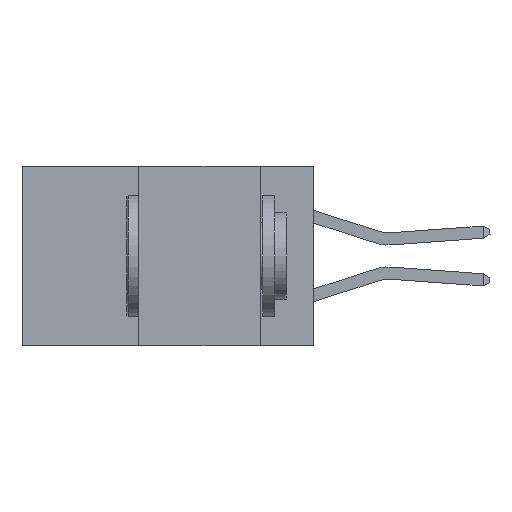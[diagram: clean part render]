
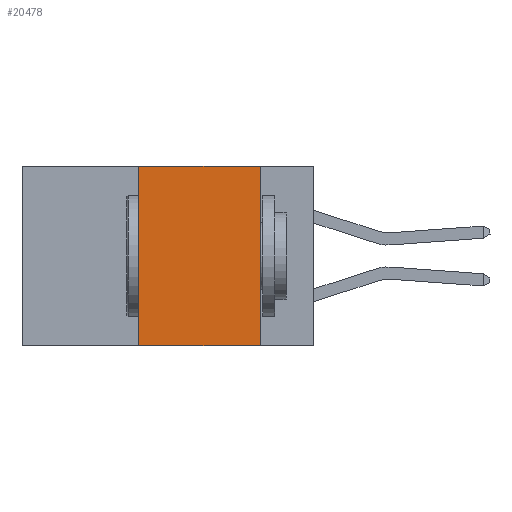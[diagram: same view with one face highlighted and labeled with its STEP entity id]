
A CAD part, left-side view. The second image highlights one B-rep face of the part: STEP entity #20478.
In plain terms, the highlighted planar face has unit normal (-1, 0, 0).
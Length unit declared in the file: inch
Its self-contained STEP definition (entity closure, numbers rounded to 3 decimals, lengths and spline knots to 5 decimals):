
#1758 = VECTOR ( 'NONE', #13715, 39.37008 ) ;
#2900 = DIRECTION ( 'NONE',  ( 0., -1., 0. ) ) ;
#2977 = CARTESIAN_POINT ( 'NONE',  ( 0., 0.36, -0.37 ) ) ;
#3043 = PLANE ( 'NONE',  #6030 ) ;
#4652 = CARTESIAN_POINT ( 'NONE',  ( 0., 0.6, 0. ) ) ;
#4727 = DIRECTION ( 'NONE',  ( 1., 0., 0. ) ) ;
#5976 = ORIENTED_EDGE ( 'NONE', *, *, #12460, .F. ) ;
#6030 = AXIS2_PLACEMENT_3D ( 'NONE', #4652, #4727, #15924 ) ;
#6099 = EDGE_CURVE ( 'NONE', #15201, #13285, #9804, .T. ) ;
#6173 = ORIENTED_EDGE ( 'NONE', *, *, #8448, .F. ) ;
#6319 = ORIENTED_EDGE ( 'NONE', *, *, #9647, .F. ) ;
#6488 = ORIENTED_EDGE ( 'NONE', *, *, #6099, .T. ) ;
#6941 = CARTESIAN_POINT ( 'NONE',  ( 0., 0.6, -0.37 ) ) ;
#7421 = DIRECTION ( 'NONE',  ( 0., 0., 1. ) ) ;
#7830 = CARTESIAN_POINT ( 'NONE',  ( 0., 0.11, -0.37 ) ) ;
#8448 = EDGE_CURVE ( 'NONE', #15726, #10926, #8983, .T. ) ;
#8568 = DIRECTION ( 'NONE',  ( 0., -1., 0. ) ) ;
#8983 = LINE ( 'NONE', #15730, #16907 ) ;
#9647 = EDGE_CURVE ( 'NONE', #15201, #15726, #11930, .T. ) ;
#9736 = CARTESIAN_POINT ( 'NONE',  ( 0., 0.11, 0. ) ) ;
#9804 = LINE ( 'NONE', #6941, #14024 ) ;
#9941 = EDGE_LOOP ( 'NONE', ( #5976, #6173, #6319, #6488 ) ) ;
#10926 = VERTEX_POINT ( 'NONE', #9736 ) ;
#11930 = LINE ( 'NONE', #18522, #19779 ) ;
#12137 = CARTESIAN_POINT ( 'NONE',  ( 0., 0.11, 0. ) ) ;
#12460 = EDGE_CURVE ( 'NONE', #10926, #13285, #13724, .T. ) ;
#13285 = VERTEX_POINT ( 'NONE', #7830 ) ;
#13715 = DIRECTION ( 'NONE',  ( 0., 0., -1. ) ) ;
#13724 = LINE ( 'NONE', #12137, #1758 ) ;
#14024 = VECTOR ( 'NONE', #8568, 39.37008 ) ;
#15168 = FACE_OUTER_BOUND ( 'NONE', #9941, .T. ) ;
#15201 = VERTEX_POINT ( 'NONE', #2977 ) ;
#15726 = VERTEX_POINT ( 'NONE', #18808 ) ;
#15730 = CARTESIAN_POINT ( 'NONE',  ( 0., 0.6, 0. ) ) ;
#15924 = DIRECTION ( 'NONE',  ( 0., 0., -1. ) ) ;
#16907 = VECTOR ( 'NONE', #2900, 39.37008 ) ;
#18522 = CARTESIAN_POINT ( 'NONE',  ( 0., 0.36, 0. ) ) ;
#18808 = CARTESIAN_POINT ( 'NONE',  ( 0., 0.36, 0. ) ) ;
#19779 = VECTOR ( 'NONE', #7421, 39.37008 ) ;
#20478 = ADVANCED_FACE ( 'NONE', ( #15168 ), #3043, .F. ) ;
